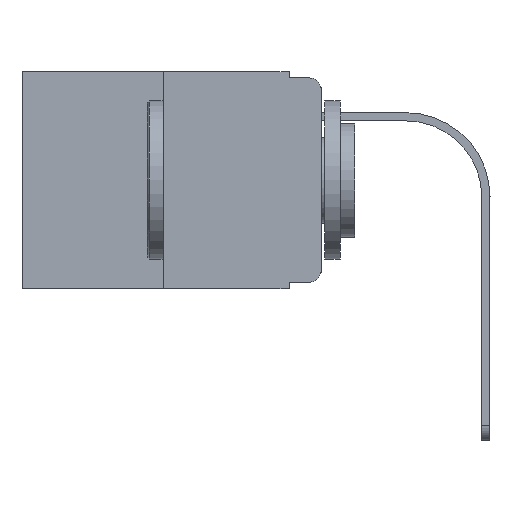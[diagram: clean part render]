
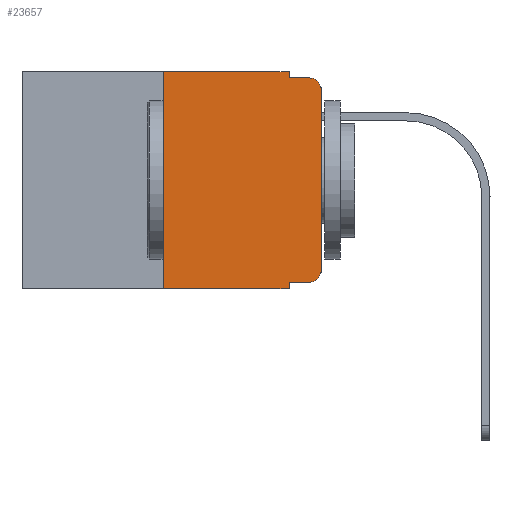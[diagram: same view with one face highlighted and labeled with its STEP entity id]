
A CAD part, left-side view. The second image highlights one B-rep face of the part: STEP entity #23657.
In plain terms, the highlighted planar face has unit normal (-1, 0, 0).
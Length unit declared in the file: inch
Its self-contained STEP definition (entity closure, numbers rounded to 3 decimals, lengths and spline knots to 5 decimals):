
#20 = EDGE_CURVE ( 'NONE', #16949, #12348, #14177, .T. ) ;
#74 = FACE_OUTER_BOUND ( 'NONE', #19877, .T. ) ;
#247 = CARTESIAN_POINT ( 'NONE',  ( 0., 0.051, 0. ) ) ;
#788 = EDGE_CURVE ( 'NONE', #12348, #4711, #4005, .T. ) ;
#1560 = VERTEX_POINT ( 'NONE', #19580 ) ;
#2102 = CARTESIAN_POINT ( 'NONE',  ( 0., 0.02, -0.313 ) ) ;
#2475 = DIRECTION ( 'NONE',  ( -1., 0., 0. ) ) ;
#3127 = AXIS2_PLACEMENT_3D ( 'NONE', #3829, #11659, #17812 ) ;
#3754 = EDGE_CURVE ( 'NONE', #14852, #24147, #19549, .T. ) ;
#3829 = CARTESIAN_POINT ( 'NONE',  ( 0., 0.473, 0. ) ) ;
#4005 = LINE ( 'NONE', #13879, #20591 ) ;
#4128 = DIRECTION ( 'NONE',  ( 0., 0., -1. ) ) ;
#4692 = VECTOR ( 'NONE', #6849, 39.37008 ) ;
#4698 = CARTESIAN_POINT ( 'NONE',  ( 0., 0., -0.03 ) ) ;
#4711 = VERTEX_POINT ( 'NONE', #12613 ) ;
#4810 = EDGE_CURVE ( 'NONE', #5484, #16949, #9025, .T. ) ;
#5098 = ORIENTED_EDGE ( 'NONE', *, *, #22464, .F. ) ;
#5151 = CARTESIAN_POINT ( 'NONE',  ( 0., 0.051, -0.01 ) ) ;
#5384 = VECTOR ( 'NONE', #20604, 39.37008 ) ;
#5484 = VERTEX_POINT ( 'NONE', #7014 ) ;
#5725 = PLANE ( 'NONE',  #3127 ) ;
#5916 = DIRECTION ( 'NONE',  ( -1., 0., 0. ) ) ;
#6799 = ORIENTED_EDGE ( 'NONE', *, *, #20, .F. ) ;
#6833 = CARTESIAN_POINT ( 'NONE',  ( 0., 0.25, 0. ) ) ;
#6849 = DIRECTION ( 'NONE',  ( 0., -1., 0. ) ) ;
#6888 = ORIENTED_EDGE ( 'NONE', *, *, #3754, .F. ) ;
#7014 = CARTESIAN_POINT ( 'NONE',  ( 0., 0.25, -0.343 ) ) ;
#7450 = VERTEX_POINT ( 'NONE', #4698 ) ;
#7589 = CARTESIAN_POINT ( 'NONE',  ( 0., 0.02, -0.01 ) ) ;
#8073 = VERTEX_POINT ( 'NONE', #7589 ) ;
#8399 = LINE ( 'NONE', #12759, #5384 ) ;
#8650 = DIRECTION ( 'NONE',  ( 0., -1., 0. ) ) ;
#8660 = AXIS2_PLACEMENT_3D ( 'NONE', #2102, #2475, #21865 ) ;
#9025 = LINE ( 'NONE', #6833, #18103 ) ;
#9355 = ORIENTED_EDGE ( 'NONE', *, *, #20537, .T. ) ;
#9416 = EDGE_CURVE ( 'NONE', #14852, #18252, #16608, .T. ) ;
#10035 = EDGE_CURVE ( 'NONE', #18252, #1560, #11952, .T. ) ;
#10585 = LINE ( 'NONE', #22267, #10626 ) ;
#10626 = VECTOR ( 'NONE', #8650, 39.37008 ) ;
#10785 = CARTESIAN_POINT ( 'NONE',  ( 0., 0.02, -0.333 ) ) ;
#11601 = AXIS2_PLACEMENT_3D ( 'NONE', #15668, #5916, #23653 ) ;
#11659 = DIRECTION ( 'NONE',  ( 1., 0., 0. ) ) ;
#11831 = DIRECTION ( 'NONE',  ( 0., 0., -1. ) ) ;
#11952 = CIRCLE ( 'NONE', #8660, 0.02 ) ;
#11998 = CIRCLE ( 'NONE', #11601, 0.02 ) ;
#12348 = VERTEX_POINT ( 'NONE', #18215 ) ;
#12613 = CARTESIAN_POINT ( 'NONE',  ( 0., 0.051, -0.01 ) ) ;
#12658 = ORIENTED_EDGE ( 'NONE', *, *, #17971, .T. ) ;
#12667 = ORIENTED_EDGE ( 'NONE', *, *, #4810, .F. ) ;
#12759 = CARTESIAN_POINT ( 'NONE',  ( 0., 0., 0. ) ) ;
#12876 = LINE ( 'NONE', #5151, #17437 ) ;
#13056 = CARTESIAN_POINT ( 'NONE',  ( 0., 0.051, -0.333 ) ) ;
#13247 = ORIENTED_EDGE ( 'NONE', *, *, #10035, .T. ) ;
#13554 = VECTOR ( 'NONE', #11831, 39.37008 ) ;
#13879 = CARTESIAN_POINT ( 'NONE',  ( 0., 0.051, 0. ) ) ;
#14177 = LINE ( 'NONE', #16356, #15296 ) ;
#14852 = VERTEX_POINT ( 'NONE', #13056 ) ;
#15296 = VECTOR ( 'NONE', #18300, 39.37008 ) ;
#15668 = CARTESIAN_POINT ( 'NONE',  ( 0., 0.02, -0.03 ) ) ;
#16343 = ORIENTED_EDGE ( 'NONE', *, *, #21180, .T. ) ;
#16356 = CARTESIAN_POINT ( 'NONE',  ( 0., 0.473, 0. ) ) ;
#16608 = LINE ( 'NONE', #24478, #4692 ) ;
#16706 = DIRECTION ( 'NONE',  ( 0., -1., 0. ) ) ;
#16949 = VERTEX_POINT ( 'NONE', #23169 ) ;
#17437 = VECTOR ( 'NONE', #16706, 39.37008 ) ;
#17812 = DIRECTION ( 'NONE',  ( 0., 0., -1. ) ) ;
#17971 = EDGE_CURVE ( 'NONE', #5484, #24147, #10585, .T. ) ;
#18103 = VECTOR ( 'NONE', #24733, 39.37008 ) ;
#18215 = CARTESIAN_POINT ( 'NONE',  ( 0., 0.051, 0. ) ) ;
#18252 = VERTEX_POINT ( 'NONE', #10785 ) ;
#18300 = DIRECTION ( 'NONE',  ( 0., -1., 0. ) ) ;
#19549 = LINE ( 'NONE', #247, #13554 ) ;
#19580 = CARTESIAN_POINT ( 'NONE',  ( 0., 0., -0.313 ) ) ;
#19877 = EDGE_LOOP ( 'NONE', ( #9355, #16343, #5098, #21693, #6799, #12667, #12658, #6888, #25244, #13247 ) ) ;
#20537 = EDGE_CURVE ( 'NONE', #1560, #7450, #8399, .T. ) ;
#20591 = VECTOR ( 'NONE', #4128, 39.37008 ) ;
#20604 = DIRECTION ( 'NONE',  ( 0., 0., 1. ) ) ;
#21180 = EDGE_CURVE ( 'NONE', #7450, #8073, #11998, .T. ) ;
#21693 = ORIENTED_EDGE ( 'NONE', *, *, #788, .F. ) ;
#21865 = DIRECTION ( 'NONE',  ( 0., 0., -1. ) ) ;
#22267 = CARTESIAN_POINT ( 'NONE',  ( 0., 0.473, -0.343 ) ) ;
#22464 = EDGE_CURVE ( 'NONE', #4711, #8073, #12876, .T. ) ;
#23169 = CARTESIAN_POINT ( 'NONE',  ( 0., 0.25, 0. ) ) ;
#23653 = DIRECTION ( 'NONE',  ( 0., 0., -1. ) ) ;
#23657 = ADVANCED_FACE ( 'NONE', ( #74 ), #5725, .F. ) ;
#24147 = VERTEX_POINT ( 'NONE', #24440 ) ;
#24440 = CARTESIAN_POINT ( 'NONE',  ( 0., 0.051, -0.343 ) ) ;
#24478 = CARTESIAN_POINT ( 'NONE',  ( 0., 0.051, -0.333 ) ) ;
#24733 = DIRECTION ( 'NONE',  ( 0., 0., 1. ) ) ;
#25244 = ORIENTED_EDGE ( 'NONE', *, *, #9416, .T. ) ;
